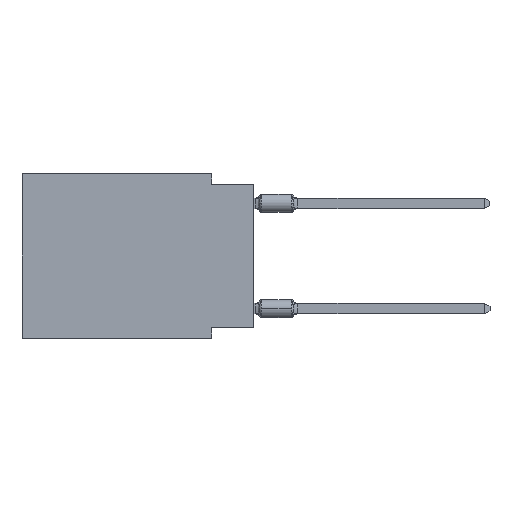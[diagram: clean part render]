
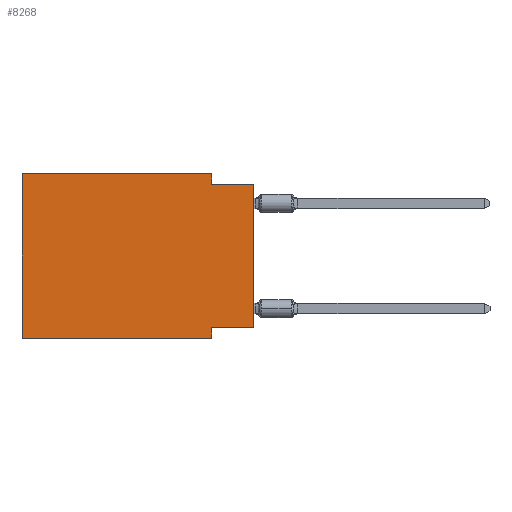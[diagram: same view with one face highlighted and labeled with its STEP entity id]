
A CAD part, left-side view. The second image highlights one B-rep face of the part: STEP entity #8268.
In plain terms, the highlighted planar face has unit normal (-1, 0, 0).
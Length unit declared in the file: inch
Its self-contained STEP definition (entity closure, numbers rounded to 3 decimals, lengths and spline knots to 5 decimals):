
#25 = EDGE_CURVE ( 'NONE', #11908, #6883, #13627, .T. ) ;
#253 = VERTEX_POINT ( 'NONE', #4326 ) ;
#357 = LINE ( 'NONE', #3914, #10475 ) ;
#940 = EDGE_CURVE ( 'NONE', #11908, #4023, #14445, .T. ) ;
#1244 = ORIENTED_EDGE ( 'NONE', *, *, #25, .F. ) ;
#1464 = EDGE_CURVE ( 'NONE', #12839, #253, #9467, .T. ) ;
#1711 = CARTESIAN_POINT ( 'NONE',  ( 0., 0., -0.365 ) ) ;
#2564 = EDGE_CURVE ( 'NONE', #9742, #4023, #6437, .T. ) ;
#2629 = VERTEX_POINT ( 'NONE', #6860 ) ;
#2712 = EDGE_CURVE ( 'NONE', #12839, #2629, #357, .T. ) ;
#2857 = DIRECTION ( 'NONE',  ( 0., -1., 0. ) ) ;
#3571 = CARTESIAN_POINT ( 'NONE',  ( 0., 0., -0.025 ) ) ;
#3914 = CARTESIAN_POINT ( 'NONE',  ( 0., 0.55, 0. ) ) ;
#3944 = ORIENTED_EDGE ( 'NONE', *, *, #940, .T. ) ;
#4023 = VERTEX_POINT ( 'NONE', #12359 ) ;
#4029 = ORIENTED_EDGE ( 'NONE', *, *, #13483, .F. ) ;
#4076 = CARTESIAN_POINT ( 'NONE',  ( 0., 0.55, -0.39 ) ) ;
#4326 = CARTESIAN_POINT ( 'NONE',  ( 0., 0.1, -0.39 ) ) ;
#4541 = ORIENTED_EDGE ( 'NONE', *, *, #2564, .F. ) ;
#4550 = CARTESIAN_POINT ( 'NONE',  ( 0., 0.1, -0.365 ) ) ;
#4588 = DIRECTION ( 'NONE',  ( 0., 0., -1. ) ) ;
#4691 = VECTOR ( 'NONE', #15132, 39.37008 ) ;
#4927 = VECTOR ( 'NONE', #7480, 39.37008 ) ;
#4947 = CARTESIAN_POINT ( 'NONE',  ( 0., 0.1, -0.025 ) ) ;
#5520 = ORIENTED_EDGE ( 'NONE', *, *, #1464, .T. ) ;
#6055 = CARTESIAN_POINT ( 'NONE',  ( 0., 0.55, 0. ) ) ;
#6143 = EDGE_CURVE ( 'NONE', #10517, #9742, #16489, .T. ) ;
#6437 = LINE ( 'NONE', #3571, #7156 ) ;
#6860 = CARTESIAN_POINT ( 'NONE',  ( 0., 0.55, 0. ) ) ;
#6883 = VERTEX_POINT ( 'NONE', #4550 ) ;
#7018 = DIRECTION ( 'NONE',  ( 0., 1., 0. ) ) ;
#7144 = LINE ( 'NONE', #15222, #4691 ) ;
#7156 = VECTOR ( 'NONE', #11469, 39.37008 ) ;
#7450 = DIRECTION ( 'NONE',  ( 1., 0., 0. ) ) ;
#7480 = DIRECTION ( 'NONE',  ( 0., 0., -1. ) ) ;
#7635 = CARTESIAN_POINT ( 'NONE',  ( 0., 0.55, -0.39 ) ) ;
#7977 = VECTOR ( 'NONE', #10105, 39.37008 ) ;
#8075 = VECTOR ( 'NONE', #4588, 39.37008 ) ;
#8268 = ADVANCED_FACE ( 'NONE', ( #12746 ), #13973, .F. ) ;
#9336 = EDGE_LOOP ( 'NONE', ( #3944, #4541, #13688, #4029, #16248, #5520, #16544, #1244 ) ) ;
#9467 = LINE ( 'NONE', #4076, #11797 ) ;
#9623 = EDGE_CURVE ( 'NONE', #6883, #253, #15374, .T. ) ;
#9742 = VERTEX_POINT ( 'NONE', #4947 ) ;
#10105 = DIRECTION ( 'NONE',  ( 0., 0., 1. ) ) ;
#10475 = VECTOR ( 'NONE', #14508, 39.37008 ) ;
#10517 = VERTEX_POINT ( 'NONE', #14695 ) ;
#11447 = CARTESIAN_POINT ( 'NONE',  ( 0., 0.1, 0. ) ) ;
#11469 = DIRECTION ( 'NONE',  ( 0., -1., 0. ) ) ;
#11634 = VECTOR ( 'NONE', #7018, 39.37008 ) ;
#11747 = CARTESIAN_POINT ( 'NONE',  ( 0., 0., 0. ) ) ;
#11797 = VECTOR ( 'NONE', #2857, 39.37008 ) ;
#11908 = VERTEX_POINT ( 'NONE', #15239 ) ;
#12359 = CARTESIAN_POINT ( 'NONE',  ( 0., 0., -0.025 ) ) ;
#12746 = FACE_OUTER_BOUND ( 'NONE', #9336, .T. ) ;
#12795 = AXIS2_PLACEMENT_3D ( 'NONE', #6055, #7450, #14141 ) ;
#12839 = VERTEX_POINT ( 'NONE', #7635 ) ;
#13483 = EDGE_CURVE ( 'NONE', #2629, #10517, #7144, .T. ) ;
#13627 = LINE ( 'NONE', #1711, #11634 ) ;
#13688 = ORIENTED_EDGE ( 'NONE', *, *, #6143, .F. ) ;
#13973 = PLANE ( 'NONE',  #12795 ) ;
#13995 = CARTESIAN_POINT ( 'NONE',  ( 0., 0.1, -0.39 ) ) ;
#14141 = DIRECTION ( 'NONE',  ( 0., 0., -1. ) ) ;
#14445 = LINE ( 'NONE', #11747, #7977 ) ;
#14508 = DIRECTION ( 'NONE',  ( 0., 0., 1. ) ) ;
#14695 = CARTESIAN_POINT ( 'NONE',  ( 0., 0.1, 0. ) ) ;
#15132 = DIRECTION ( 'NONE',  ( 0., -1., 0. ) ) ;
#15222 = CARTESIAN_POINT ( 'NONE',  ( 0., 0.55, 0. ) ) ;
#15239 = CARTESIAN_POINT ( 'NONE',  ( 0., 0., -0.365 ) ) ;
#15374 = LINE ( 'NONE', #13995, #4927 ) ;
#16248 = ORIENTED_EDGE ( 'NONE', *, *, #2712, .F. ) ;
#16489 = LINE ( 'NONE', #11447, #8075 ) ;
#16544 = ORIENTED_EDGE ( 'NONE', *, *, #9623, .F. ) ;
